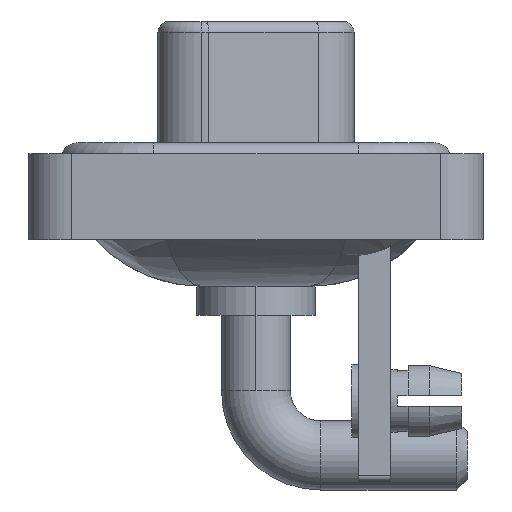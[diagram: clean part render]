
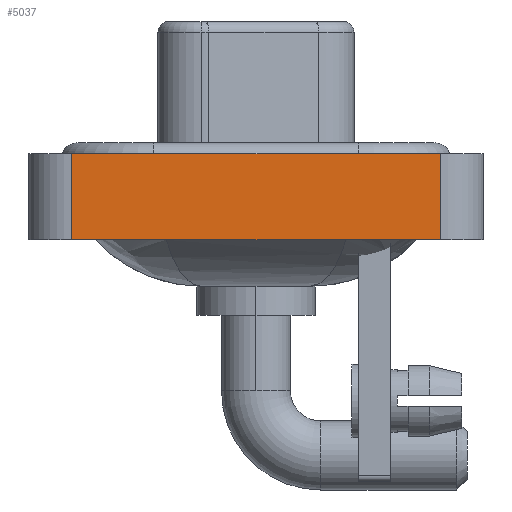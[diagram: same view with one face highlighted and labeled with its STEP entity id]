
A CAD part, left-side view. The second image highlights one B-rep face of the part: STEP entity #5037.
In plain terms, the highlighted planar face has unit normal (-1, 0, 0).
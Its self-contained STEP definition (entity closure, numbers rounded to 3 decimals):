
#756 = VERTEX_POINT ( 'NONE', #9435 ) ;
#1031 = DIRECTION ( 'NONE',  ( 0., 0., 1. ) ) ;
#1645 = DIRECTION ( 'NONE',  ( -1., 0., 0. ) ) ;
#3105 = ORIENTED_EDGE ( 'NONE', *, *, #18526, .F. ) ;
#3630 = VERTEX_POINT ( 'NONE', #6505 ) ;
#3889 = LINE ( 'NONE', #10216, #10906 ) ;
#4333 = EDGE_CURVE ( 'NONE', #13282, #3630, #14452, .T. ) ;
#4471 = EDGE_CURVE ( 'NONE', #10471, #3630, #3889, .T. ) ;
#5024 = CARTESIAN_POINT ( 'NONE',  ( -7.35, -8.55, -3.6 ) ) ;
#5037 = ADVANCED_FACE ( 'NONE', ( #6205 ), #12514, .T. ) ;
#5161 = CARTESIAN_POINT ( 'NONE',  ( -7.35, 8.55, 0.4 ) ) ;
#6205 = FACE_OUTER_BOUND ( 'NONE', #10060, .T. ) ;
#6399 = ORIENTED_EDGE ( 'NONE', *, *, #7833, .T. ) ;
#6505 = CARTESIAN_POINT ( 'NONE',  ( -7.35, -8.55, 0.4 ) ) ;
#6686 = ORIENTED_EDGE ( 'NONE', *, *, #4333, .T. ) ;
#7833 = EDGE_CURVE ( 'NONE', #756, #13282, #19652, .T. ) ;
#8453 = DIRECTION ( 'NONE',  ( 0., 0., 1. ) ) ;
#9435 = CARTESIAN_POINT ( 'NONE',  ( -7.35, 8.55, -3.6 ) ) ;
#9611 = AXIS2_PLACEMENT_3D ( 'NONE', #18835, #1645, #12615 ) ;
#9912 = VECTOR ( 'NONE', #8453, 1000. ) ;
#10060 = EDGE_LOOP ( 'NONE', ( #6686, #14079, #3105, #6399 ) ) ;
#10216 = CARTESIAN_POINT ( 'NONE',  ( -7.35, -8.55, 0.4 ) ) ;
#10444 = LINE ( 'NONE', #17045, #18576 ) ;
#10471 = VERTEX_POINT ( 'NONE', #5161 ) ;
#10906 = VECTOR ( 'NONE', #15187, 1000. ) ;
#12514 = PLANE ( 'NONE',  #9611 ) ;
#12615 = DIRECTION ( 'NONE',  ( 0., 0., 1. ) ) ;
#13023 = DIRECTION ( 'NONE',  ( 0., -1., 0. ) ) ;
#13282 = VERTEX_POINT ( 'NONE', #18022 ) ;
#14079 = ORIENTED_EDGE ( 'NONE', *, *, #4471, .F. ) ;
#14452 = LINE ( 'NONE', #5024, #9912 ) ;
#15004 = VECTOR ( 'NONE', #13023, 1000. ) ;
#15187 = DIRECTION ( 'NONE',  ( 0., -1., 0. ) ) ;
#17045 = CARTESIAN_POINT ( 'NONE',  ( -7.35, 8.55, -3.6 ) ) ;
#18022 = CARTESIAN_POINT ( 'NONE',  ( -7.35, -8.55, -3.6 ) ) ;
#18096 = CARTESIAN_POINT ( 'NONE',  ( -7.35, -8.55, -3.6 ) ) ;
#18526 = EDGE_CURVE ( 'NONE', #756, #10471, #10444, .T. ) ;
#18576 = VECTOR ( 'NONE', #1031, 1000. ) ;
#18835 = CARTESIAN_POINT ( 'NONE',  ( -7.35, -8.55, -3.6 ) ) ;
#19652 = LINE ( 'NONE', #18096, #15004 ) ;
